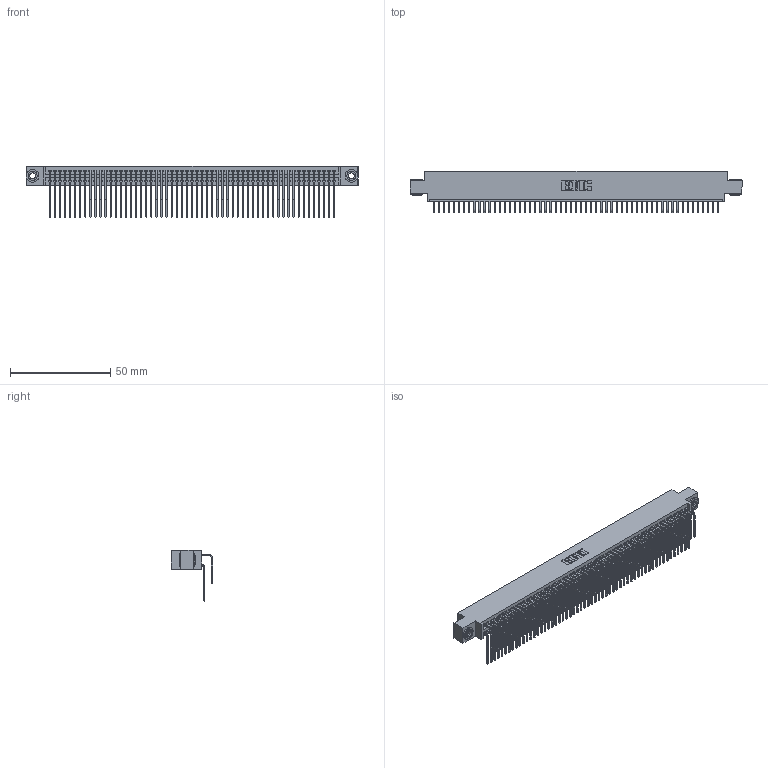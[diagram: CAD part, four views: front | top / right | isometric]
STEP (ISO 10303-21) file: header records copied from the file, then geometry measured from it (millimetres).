
FILE_DESCRIPTION (( 'STEP AP203' ), '1' );
FILE_NAME ('395-114-559-803.STEP', '2019-10-27T19:33:40', ( '' ), ( '' ), 'SwSTEP 2.0', 'SolidWorks 2016', '' );
FILE_SCHEMA (( 'CONFIG_CONTROL_DESIGN' ));
Length unit declared in the file: inch
Products named in the file (5): 345 Part_0.170 Offset - 0.156 Dia-TH; 345-292-001_558 559 Tail - 1; 345-292-001_559 Tail - 2; 345-250-002_345-250-002-102; 395-114-559-803
Assembly tree (117 placements, depth 2):
  395-114-559-803
    345 Part_0.170 Offset - 0.156 Dia-TH
    345-292-001_558 559 Tail - 1  x57
    345-292-001_559 Tail - 2  x57
    345-250-002_345-250-002-102  x2
Bounding box: 165.99 x 20.56 x 25.53 mm (x, y, z)
Volume: 16827.2 mm3; surface area: 28604.8 mm2
Topology: 117 solids, 117 shells, 6096 faces, 18099 edges, 11910 vertices
Faces by surface type: plane 4084, cylinder 2004, cone 8
Entity records: 45138 total; most frequent: CARTESIAN_POINT 7574, ORIENTED_EDGE 7450, DIRECTION 6663, EDGE_CURVE 3725, LINE 3301, VECTOR 3301, VERTEX_POINT 2478, AXIS2_PLACEMENT_3D 1681
